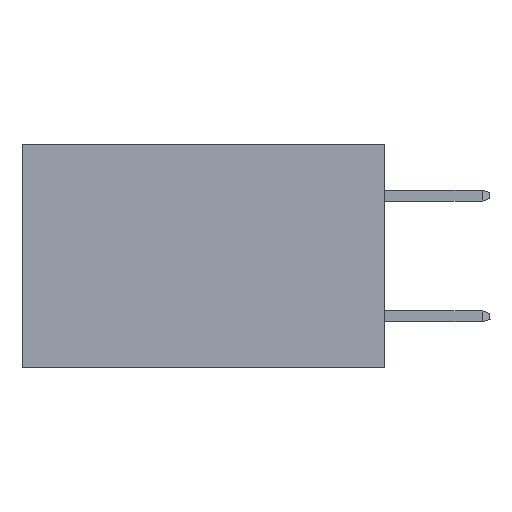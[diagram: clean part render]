
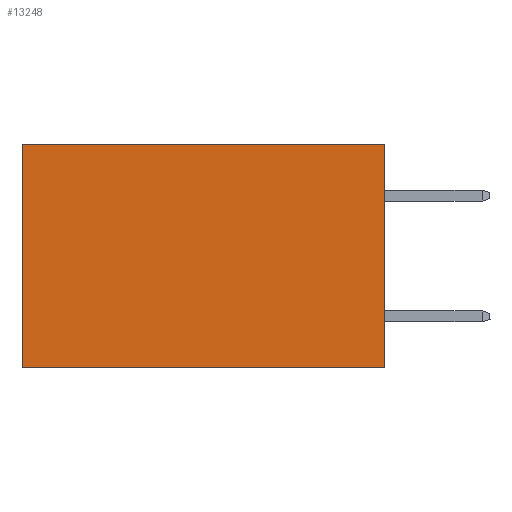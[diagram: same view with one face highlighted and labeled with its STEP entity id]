
A CAD part, left-side view. The second image highlights one B-rep face of the part: STEP entity #13248.
In plain terms, the highlighted planar face has unit normal (-1, 0, 0).
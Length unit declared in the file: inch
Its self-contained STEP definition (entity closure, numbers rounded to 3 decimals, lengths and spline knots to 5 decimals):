
#67 = ORIENTED_EDGE ( 'NONE', *, *, #13201, .T. ) ;
#2038 = EDGE_LOOP ( 'NONE', ( #67, #15562, #7826, #10369 ) ) ;
#2537 = VECTOR ( 'NONE', #3995, 39.37008 ) ;
#3046 = VECTOR ( 'NONE', #11269, 39.37008 ) ;
#3129 = EDGE_CURVE ( 'NONE', #9249, #10719, #19296, .T. ) ;
#3167 = CARTESIAN_POINT ( 'NONE',  ( 0.2615, 0.6, 0. ) ) ;
#3523 = LINE ( 'NONE', #9749, #3046 ) ;
#3858 = LINE ( 'NONE', #8345, #6408 ) ;
#3995 = DIRECTION ( 'NONE',  ( 0., 1., 0. ) ) ;
#4117 = EDGE_CURVE ( 'NONE', #14853, #7564, #14068, .T. ) ;
#4250 = CARTESIAN_POINT ( 'NONE',  ( 0.2615, 0., -0.37 ) ) ;
#4378 = CARTESIAN_POINT ( 'NONE',  ( 0.2615, 0., 0. ) ) ;
#5090 = CARTESIAN_POINT ( 'NONE',  ( 0.2615, 0., -0.37 ) ) ;
#5283 = CARTESIAN_POINT ( 'NONE',  ( 0.2615, 0., -0.37 ) ) ;
#6408 = VECTOR ( 'NONE', #12920, 39.37008 ) ;
#6817 = DIRECTION ( 'NONE',  ( 1., 0., 0. ) ) ;
#7564 = VERTEX_POINT ( 'NONE', #9519 ) ;
#7826 = ORIENTED_EDGE ( 'NONE', *, *, #17004, .F. ) ;
#8175 = VECTOR ( 'NONE', #17164, 39.37008 ) ;
#8345 = CARTESIAN_POINT ( 'NONE',  ( 0.2615, 0., -0.37 ) ) ;
#9249 = VERTEX_POINT ( 'NONE', #4378 ) ;
#9519 = CARTESIAN_POINT ( 'NONE',  ( 0.2615, 0.6, -0.37 ) ) ;
#9749 = CARTESIAN_POINT ( 'NONE',  ( 0.2615, 0.6, -0.37 ) ) ;
#10369 = ORIENTED_EDGE ( 'NONE', *, *, #3129, .T. ) ;
#10719 = VERTEX_POINT ( 'NONE', #3167 ) ;
#11269 = DIRECTION ( 'NONE',  ( 0., 0., -1. ) ) ;
#12920 = DIRECTION ( 'NONE',  ( 0., 0., -1. ) ) ;
#13201 = EDGE_CURVE ( 'NONE', #10719, #7564, #3523, .T. ) ;
#13248 = ADVANCED_FACE ( 'NONE', ( #13648 ), #15912, .F. ) ;
#13648 = FACE_OUTER_BOUND ( 'NONE', #2038, .T. ) ;
#14068 = LINE ( 'NONE', #4250, #2537 ) ;
#14853 = VERTEX_POINT ( 'NONE', #5090 ) ;
#15297 = AXIS2_PLACEMENT_3D ( 'NONE', #5283, #6817, #17422 ) ;
#15562 = ORIENTED_EDGE ( 'NONE', *, *, #4117, .F. ) ;
#15912 = PLANE ( 'NONE',  #15297 ) ;
#17004 = EDGE_CURVE ( 'NONE', #9249, #14853, #3858, .T. ) ;
#17064 = CARTESIAN_POINT ( 'NONE',  ( 0.2615, 0., 0. ) ) ;
#17164 = DIRECTION ( 'NONE',  ( 0., 1., 0. ) ) ;
#17422 = DIRECTION ( 'NONE',  ( 0., 0., -1. ) ) ;
#19296 = LINE ( 'NONE', #17064, #8175 ) ;
